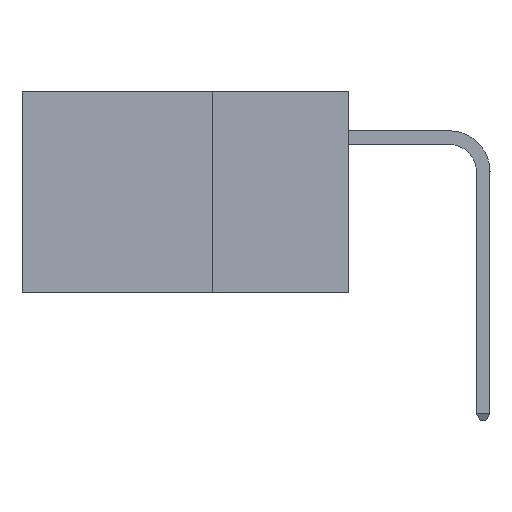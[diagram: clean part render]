
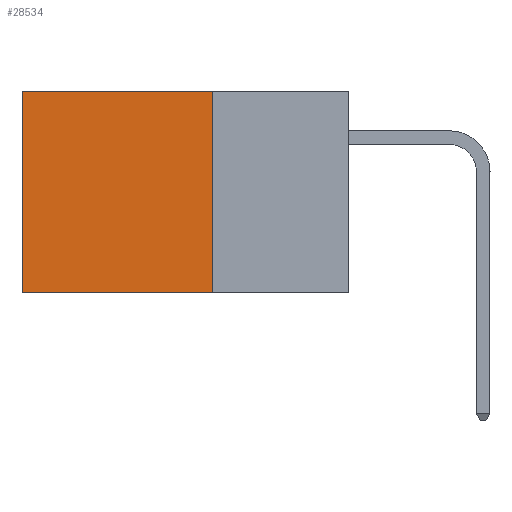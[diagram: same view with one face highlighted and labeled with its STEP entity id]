
A CAD part, left-side view. The second image highlights one B-rep face of the part: STEP entity #28534.
In plain terms, the highlighted planar face has unit normal (-1, 0, 0).
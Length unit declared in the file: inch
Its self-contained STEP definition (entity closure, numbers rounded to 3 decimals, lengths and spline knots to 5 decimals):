
#206 = CARTESIAN_POINT ( 'NONE',  ( 0.2875, 0.25, 0. ) ) ;
#4994 = AXIS2_PLACEMENT_3D ( 'NONE', #206, #32146, #14909 ) ;
#5140 = ORIENTED_EDGE ( 'NONE', *, *, #30524, .F. ) ;
#6087 = VERTEX_POINT ( 'NONE', #13406 ) ;
#7105 = FACE_OUTER_BOUND ( 'NONE', #23219, .T. ) ;
#7304 = ORIENTED_EDGE ( 'NONE', *, *, #21461, .F. ) ;
#7404 = CARTESIAN_POINT ( 'NONE',  ( 0.2875, 0.25, -0.37 ) ) ;
#9212 = ORIENTED_EDGE ( 'NONE', *, *, #10476, .T. ) ;
#9808 = EDGE_CURVE ( 'NONE', #37431, #12781, #20325, .T. ) ;
#10476 = EDGE_CURVE ( 'NONE', #6087, #37431, #33203, .T. ) ;
#12781 = VERTEX_POINT ( 'NONE', #25489 ) ;
#13000 = VECTOR ( 'NONE', #17357, 39.37008 ) ;
#13406 = CARTESIAN_POINT ( 'NONE',  ( 0.2875, 0.25, 0. ) ) ;
#13876 = VECTOR ( 'NONE', #24900, 39.37008 ) ;
#14434 = CARTESIAN_POINT ( 'NONE',  ( 0.2875, 0.25, 0. ) ) ;
#14909 = DIRECTION ( 'NONE',  ( 0., 0., -1. ) ) ;
#15854 = CARTESIAN_POINT ( 'NONE',  ( 0.2875, 0.6, 0. ) ) ;
#17274 = CARTESIAN_POINT ( 'NONE',  ( 0.2875, 0.6, 0. ) ) ;
#17357 = DIRECTION ( 'NONE',  ( 0., 1., 0. ) ) ;
#20325 = LINE ( 'NONE', #17274, #27007 ) ;
#21461 = EDGE_CURVE ( 'NONE', #6087, #32180, #36352, .T. ) ;
#22111 = VECTOR ( 'NONE', #31541, 39.37008 ) ;
#23219 = EDGE_LOOP ( 'NONE', ( #25016, #5140, #7304, #9212 ) ) ;
#24900 = DIRECTION ( 'NONE',  ( 0., 1., 0. ) ) ;
#25016 = ORIENTED_EDGE ( 'NONE', *, *, #9808, .T. ) ;
#25489 = CARTESIAN_POINT ( 'NONE',  ( 0.2875, 0.6, -0.37 ) ) ;
#26277 = CARTESIAN_POINT ( 'NONE',  ( 0.2875, 0.25, -0.37 ) ) ;
#27007 = VECTOR ( 'NONE', #31584, 39.37008 ) ;
#28534 = ADVANCED_FACE ( 'NONE', ( #7105 ), #29286, .F. ) ;
#29192 = LINE ( 'NONE', #7404, #13876 ) ;
#29286 = PLANE ( 'NONE',  #4994 ) ;
#30524 = EDGE_CURVE ( 'NONE', #32180, #12781, #29192, .T. ) ;
#31541 = DIRECTION ( 'NONE',  ( 0., 0., -1. ) ) ;
#31584 = DIRECTION ( 'NONE',  ( 0., 0., -1. ) ) ;
#31659 = CARTESIAN_POINT ( 'NONE',  ( 0.2875, 0.25, 0. ) ) ;
#32146 = DIRECTION ( 'NONE',  ( 1., 0., 0. ) ) ;
#32180 = VERTEX_POINT ( 'NONE', #26277 ) ;
#33203 = LINE ( 'NONE', #14434, #13000 ) ;
#36352 = LINE ( 'NONE', #31659, #22111 ) ;
#37431 = VERTEX_POINT ( 'NONE', #15854 ) ;
